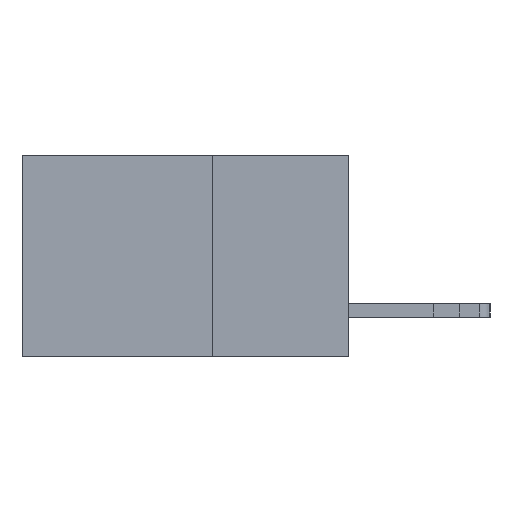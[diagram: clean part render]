
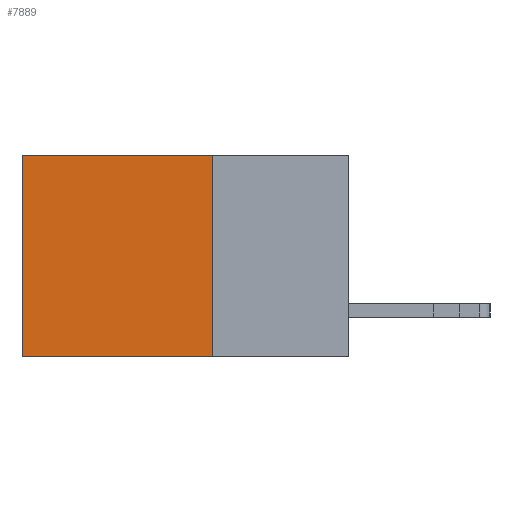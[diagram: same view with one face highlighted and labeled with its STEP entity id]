
A CAD part, left-side view. The second image highlights one B-rep face of the part: STEP entity #7889.
In plain terms, the highlighted planar face has unit normal (-1, 0, 0).
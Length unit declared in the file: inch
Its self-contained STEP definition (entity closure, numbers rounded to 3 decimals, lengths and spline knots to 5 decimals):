
#4 = FACE_OUTER_BOUND ( 'NONE', #6602, .T. ) ;
#58 = DIRECTION ( 'NONE',  ( 0., 1., 0. ) ) ;
#316 = DIRECTION ( 'NONE',  ( 0., 0., -1. ) ) ;
#396 = EDGE_CURVE ( 'NONE', #4091, #7415, #7086, .T. ) ;
#703 = VECTOR ( 'NONE', #12725, 39.37008 ) ;
#814 = CARTESIAN_POINT ( 'NONE',  ( 0.298, 0.25, 0. ) ) ;
#936 = CARTESIAN_POINT ( 'NONE',  ( 0.298, 0.25, 0. ) ) ;
#1484 = CARTESIAN_POINT ( 'NONE',  ( 0.298, 0.25, 0. ) ) ;
#1500 = VERTEX_POINT ( 'NONE', #11289 ) ;
#1868 = VERTEX_POINT ( 'NONE', #2102 ) ;
#1944 = VECTOR ( 'NONE', #316, 39.37008 ) ;
#2102 = CARTESIAN_POINT ( 'NONE',  ( 0.298, 0.6, 0. ) ) ;
#2213 = AXIS2_PLACEMENT_3D ( 'NONE', #814, #11246, #5235 ) ;
#2281 = CARTESIAN_POINT ( 'NONE',  ( 0.298, 0.25, -0.37 ) ) ;
#2441 = VECTOR ( 'NONE', #58, 39.37008 ) ;
#3138 = CARTESIAN_POINT ( 'NONE',  ( 0.298, 0.25, -0.37 ) ) ;
#4040 = ORIENTED_EDGE ( 'NONE', *, *, #9734, .T. ) ;
#4091 = VERTEX_POINT ( 'NONE', #9669 ) ;
#4569 = VECTOR ( 'NONE', #9285, 39.37008 ) ;
#5235 = DIRECTION ( 'NONE',  ( 0., 0., -1. ) ) ;
#5460 = EDGE_CURVE ( 'NONE', #7415, #1500, #13189, .T. ) ;
#5797 = CARTESIAN_POINT ( 'NONE',  ( 0.298, 0.6, 0. ) ) ;
#6602 = EDGE_LOOP ( 'NONE', ( #4040, #7576, #11950, #11483 ) ) ;
#7086 = LINE ( 'NONE', #936, #4569 ) ;
#7415 = VERTEX_POINT ( 'NONE', #2281 ) ;
#7576 = ORIENTED_EDGE ( 'NONE', *, *, #5460, .F. ) ;
#7889 = ADVANCED_FACE ( 'NONE', ( #4 ), #10304, .F. ) ;
#8955 = LINE ( 'NONE', #1484, #703 ) ;
#9285 = DIRECTION ( 'NONE',  ( 0., 0., -1. ) ) ;
#9669 = CARTESIAN_POINT ( 'NONE',  ( 0.298, 0.25, 0. ) ) ;
#9734 = EDGE_CURVE ( 'NONE', #1868, #1500, #10009, .T. ) ;
#10009 = LINE ( 'NONE', #5797, #1944 ) ;
#10109 = EDGE_CURVE ( 'NONE', #4091, #1868, #8955, .T. ) ;
#10304 = PLANE ( 'NONE',  #2213 ) ;
#11246 = DIRECTION ( 'NONE',  ( 1., 0., 0. ) ) ;
#11289 = CARTESIAN_POINT ( 'NONE',  ( 0.298, 0.6, -0.37 ) ) ;
#11483 = ORIENTED_EDGE ( 'NONE', *, *, #10109, .T. ) ;
#11950 = ORIENTED_EDGE ( 'NONE', *, *, #396, .F. ) ;
#12725 = DIRECTION ( 'NONE',  ( 0., 1., 0. ) ) ;
#13189 = LINE ( 'NONE', #3138, #2441 ) ;
